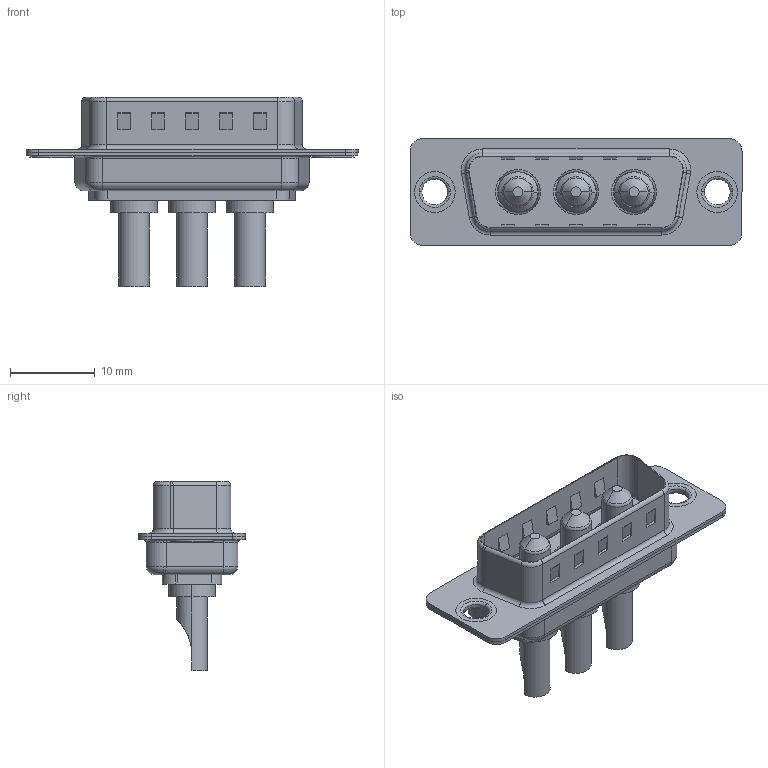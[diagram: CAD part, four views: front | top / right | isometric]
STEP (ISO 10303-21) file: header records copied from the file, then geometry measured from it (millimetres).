
FILE_DESCRIPTION (( 'STEP AP203' ), '1' );
FILE_NAME ('627-3W3-222-2N1.STEP', '2019-05-24T12:49:50', ( '' ), ( '' ), 'SwSTEP 2.0', 'SolidWorks 2016', '' );
FILE_SCHEMA (( 'CONFIG_CONTROL_DESIGN' ));
Length unit declared in the file: millimetre
Products named in the file (6): 627Combo Thru Hole Rivet; Power Pin_20A SC; 627-3W3-222-2N1; 627Combo Housing_3W3; 627Combo Shell Rear_15 Contacts; 627Combo Shell Front_15 Contacts
Assembly tree (8 placements, depth 2):
  627-3W3-222-2N1
    627Combo Housing_3W3
    627Combo Shell Rear_15 Contacts
    627Combo Shell Front_15 Contacts
    627Combo Thru Hole Rivet  x2
    Power Pin_20A SC  x3
Bounding box: 39.15 x 12.6 x 22.3 mm (x, y, z)
Volume: 2009.5 mm3; surface area: 4808.6 mm2
Topology: 11 solids, 11 shells, 452 faces, 1081 edges, 665 vertices
Faces by surface type: cylinder 183, plane 178, torus 64, cone 21, bspline 6
Entity records: 11210 total; most frequent: CARTESIAN_POINT 1932, DIRECTION 1903, ORIENTED_EDGE 1714, EDGE_CURVE 857, AXIS2_PLACEMENT_3D 710, VERTEX_POINT 535, VECTOR 483, LINE 483
